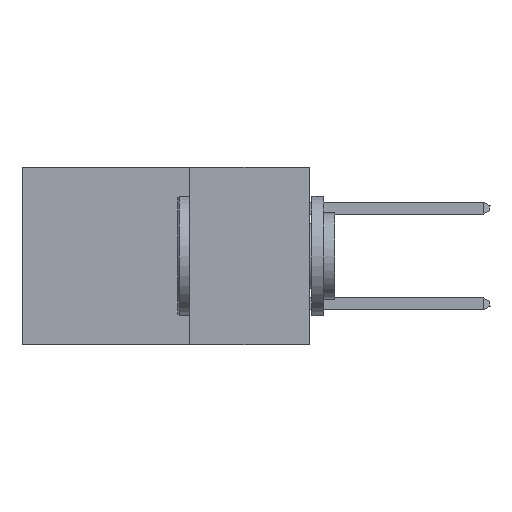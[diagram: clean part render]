
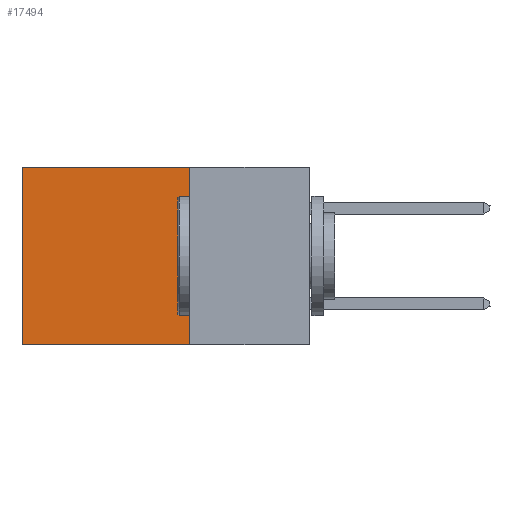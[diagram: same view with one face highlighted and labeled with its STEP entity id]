
A CAD part, left-side view. The second image highlights one B-rep face of the part: STEP entity #17494.
In plain terms, the highlighted planar face has unit normal (-1, 0, 0).
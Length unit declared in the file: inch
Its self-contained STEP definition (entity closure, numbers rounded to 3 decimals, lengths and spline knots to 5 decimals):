
#655 = CARTESIAN_POINT ( 'NONE',  ( 0.2875, 0.25, 0. ) ) ;
#1585 = EDGE_CURVE ( 'NONE', #34822, #25173, #21345, .T. ) ;
#2530 = VERTEX_POINT ( 'NONE', #19165 ) ;
#5095 = VECTOR ( 'NONE', #20486, 39.37008 ) ;
#5120 = CARTESIAN_POINT ( 'NONE',  ( 0.2875, 0.6, 0. ) ) ;
#5578 = VECTOR ( 'NONE', #11701, 39.37008 ) ;
#6878 = EDGE_CURVE ( 'NONE', #28811, #25173, #28231, .T. ) ;
#7204 = ORIENTED_EDGE ( 'NONE', *, *, #7357, .F. ) ;
#7206 = CARTESIAN_POINT ( 'NONE',  ( 0.2875, 0.25, -0.37 ) ) ;
#7240 = CARTESIAN_POINT ( 'NONE',  ( 0.2875, 0.6, 0. ) ) ;
#7357 = EDGE_CURVE ( 'NONE', #2530, #28811, #19769, .T. ) ;
#8292 = AXIS2_PLACEMENT_3D ( 'NONE', #8612, #14002, #22086 ) ;
#8612 = CARTESIAN_POINT ( 'NONE',  ( 0.2875, 0.25, 0. ) ) ;
#11701 = DIRECTION ( 'NONE',  ( 0., 1., 0. ) ) ;
#11756 = ORIENTED_EDGE ( 'NONE', *, *, #23435, .T. ) ;
#14002 = DIRECTION ( 'NONE',  ( 1., 0., 0. ) ) ;
#17494 = ADVANCED_FACE ( 'NONE', ( #30283 ), #30183, .F. ) ;
#17551 = CARTESIAN_POINT ( 'NONE',  ( 0.2875, 0.25, -0.37 ) ) ;
#19165 = CARTESIAN_POINT ( 'NONE',  ( 0.2875, 0.25, 0. ) ) ;
#19769 = LINE ( 'NONE', #19923, #21053 ) ;
#19923 = CARTESIAN_POINT ( 'NONE',  ( 0.2875, 0.25, 0. ) ) ;
#20486 = DIRECTION ( 'NONE',  ( 0., 1., 0. ) ) ;
#21053 = VECTOR ( 'NONE', #27802, 39.37008 ) ;
#21160 = LINE ( 'NONE', #655, #5578 ) ;
#21345 = LINE ( 'NONE', #5120, #33991 ) ;
#22086 = DIRECTION ( 'NONE',  ( 0., 0., -1. ) ) ;
#23435 = EDGE_CURVE ( 'NONE', #2530, #34822, #21160, .T. ) ;
#23910 = DIRECTION ( 'NONE',  ( 0., 0., -1. ) ) ;
#25173 = VERTEX_POINT ( 'NONE', #26441 ) ;
#26182 = ORIENTED_EDGE ( 'NONE', *, *, #6878, .F. ) ;
#26441 = CARTESIAN_POINT ( 'NONE',  ( 0.2875, 0.6, -0.37 ) ) ;
#27802 = DIRECTION ( 'NONE',  ( 0., 0., -1. ) ) ;
#28231 = LINE ( 'NONE', #17551, #5095 ) ;
#28811 = VERTEX_POINT ( 'NONE', #7206 ) ;
#29231 = ORIENTED_EDGE ( 'NONE', *, *, #1585, .T. ) ;
#30183 = PLANE ( 'NONE',  #8292 ) ;
#30283 = FACE_OUTER_BOUND ( 'NONE', #33766, .T. ) ;
#33766 = EDGE_LOOP ( 'NONE', ( #29231, #26182, #7204, #11756 ) ) ;
#33991 = VECTOR ( 'NONE', #23910, 39.37008 ) ;
#34822 = VERTEX_POINT ( 'NONE', #7240 ) ;
